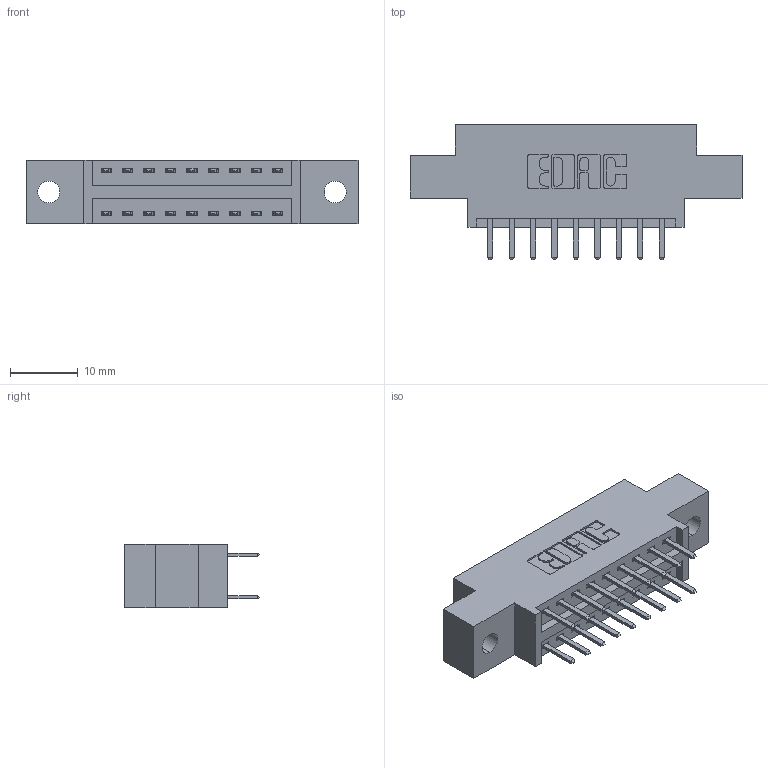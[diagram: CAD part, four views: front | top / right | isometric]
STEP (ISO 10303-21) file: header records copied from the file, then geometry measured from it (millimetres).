
FILE_DESCRIPTION (( 'STEP AP203' ), '1' );
FILE_NAME ('396-018-520-802.STEP', '2019-11-01T17:44:29', ( '' ), ( '' ), 'SwSTEP 2.0', 'SolidWorks 2016', '' );
FILE_SCHEMA (( 'CONFIG_CONTROL_DESIGN' ));
Length unit declared in the file: inch
Products named in the file (3): 396-018-520-802; 346 Part_0.170 Offset - 0.128 Dia; 345-292-001_345-293-120
Assembly tree (19 placements, depth 2):
  396-018-520-802
    346 Part_0.170 Offset - 0.128 Dia
    345-292-001_345-293-120  x18
Bounding box: 49.15 x 20.02 x 9.4 mm (x, y, z)
Volume: 4337.1 mm3; surface area: 5334.8 mm2
Topology: 19 solids, 19 shells, 1134 faces, 3275 edges, 2134 vertices
Faces by surface type: plane 746, cylinder 388
Entity records: 10565 total; most frequent: CARTESIAN_POINT 1800, ORIENTED_EDGE 1722, DIRECTION 1625, EDGE_CURVE 861, VECTOR 689, LINE 689, VERTEX_POINT 570, AXIS2_PLACEMENT_3D 468
